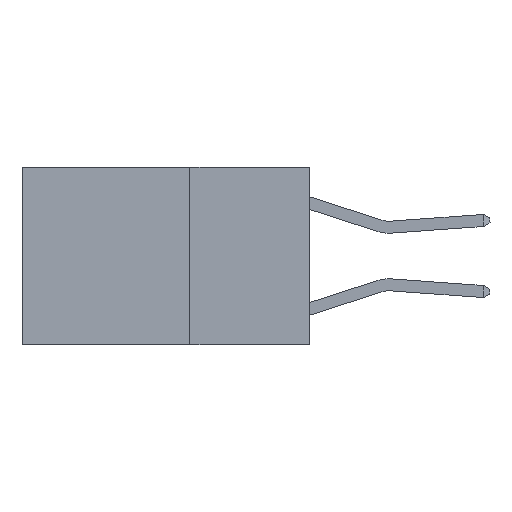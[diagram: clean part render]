
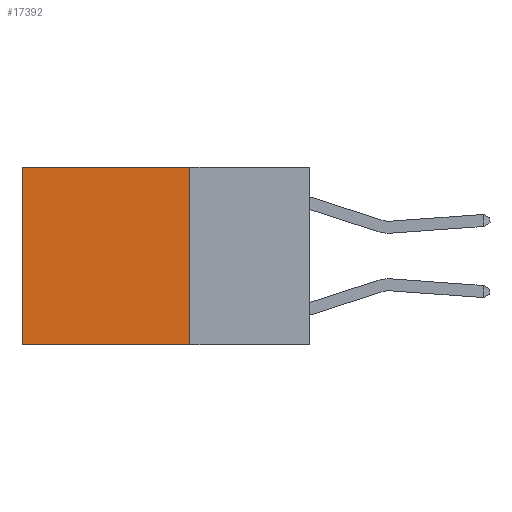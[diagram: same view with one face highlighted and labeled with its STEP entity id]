
A CAD part, left-side view. The second image highlights one B-rep face of the part: STEP entity #17392.
In plain terms, the highlighted planar face has unit normal (-1, 0, 0).
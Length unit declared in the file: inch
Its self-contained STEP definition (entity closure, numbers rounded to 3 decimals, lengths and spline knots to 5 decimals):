
#1124 = ORIENTED_EDGE ( 'NONE', *, *, #5699, .T. ) ;
#2429 = LINE ( 'NONE', #13835, #23933 ) ;
#3128 = DIRECTION ( 'NONE',  ( 0., 0., -1. ) ) ;
#3898 = VECTOR ( 'NONE', #3128, 39.37008 ) ;
#4144 = VERTEX_POINT ( 'NONE', #23446 ) ;
#5242 = VERTEX_POINT ( 'NONE', #10549 ) ;
#5699 = EDGE_CURVE ( 'NONE', #19000, #4144, #2429, .T. ) ;
#5765 = CARTESIAN_POINT ( 'NONE',  ( 0.2625, 0.6, -0.37 ) ) ;
#6692 = CARTESIAN_POINT ( 'NONE',  ( 0.2625, 0.6, 0. ) ) ;
#7028 = PLANE ( 'NONE',  #11891 ) ;
#7262 = VERTEX_POINT ( 'NONE', #5765 ) ;
#7540 = EDGE_CURVE ( 'NONE', #19000, #5242, #14363, .T. ) ;
#7858 = DIRECTION ( 'NONE',  ( 0., 1., 0. ) ) ;
#9335 = EDGE_LOOP ( 'NONE', ( #18151, #21289, #12274, #1124 ) ) ;
#9344 = LINE ( 'NONE', #6692, #3898 ) ;
#10152 = CARTESIAN_POINT ( 'NONE',  ( 0.2625, 0.25, 0. ) ) ;
#10549 = CARTESIAN_POINT ( 'NONE',  ( 0.2625, 0.25, -0.37 ) ) ;
#11068 = DIRECTION ( 'NONE',  ( 0., 0., -1. ) ) ;
#11291 = FACE_OUTER_BOUND ( 'NONE', #9335, .T. ) ;
#11446 = CARTESIAN_POINT ( 'NONE',  ( 0.2625, 0.25, 0. ) ) ;
#11891 = AXIS2_PLACEMENT_3D ( 'NONE', #18925, #23074, #11068 ) ;
#12146 = LINE ( 'NONE', #25413, #13375 ) ;
#12274 = ORIENTED_EDGE ( 'NONE', *, *, #7540, .F. ) ;
#13375 = VECTOR ( 'NONE', #19715, 39.37008 ) ;
#13835 = CARTESIAN_POINT ( 'NONE',  ( 0.2625, 0.25, 0. ) ) ;
#14363 = LINE ( 'NONE', #10152, #25109 ) ;
#17392 = ADVANCED_FACE ( 'NONE', ( #11291 ), #7028, .F. ) ;
#18151 = ORIENTED_EDGE ( 'NONE', *, *, #18719, .T. ) ;
#18719 = EDGE_CURVE ( 'NONE', #4144, #7262, #9344, .T. ) ;
#18925 = CARTESIAN_POINT ( 'NONE',  ( 0.2625, 0.25, 0. ) ) ;
#19000 = VERTEX_POINT ( 'NONE', #11446 ) ;
#19715 = DIRECTION ( 'NONE',  ( 0., 1., 0. ) ) ;
#20181 = DIRECTION ( 'NONE',  ( 0., 0., -1. ) ) ;
#21289 = ORIENTED_EDGE ( 'NONE', *, *, #22462, .F. ) ;
#22462 = EDGE_CURVE ( 'NONE', #5242, #7262, #12146, .T. ) ;
#23074 = DIRECTION ( 'NONE',  ( 1., 0., 0. ) ) ;
#23446 = CARTESIAN_POINT ( 'NONE',  ( 0.2625, 0.6, 0. ) ) ;
#23933 = VECTOR ( 'NONE', #7858, 39.37008 ) ;
#25109 = VECTOR ( 'NONE', #20181, 39.37008 ) ;
#25413 = CARTESIAN_POINT ( 'NONE',  ( 0.2625, 0.25, -0.37 ) ) ;
